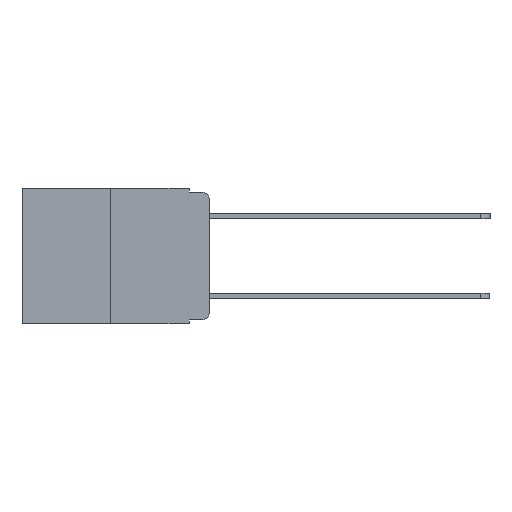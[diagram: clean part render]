
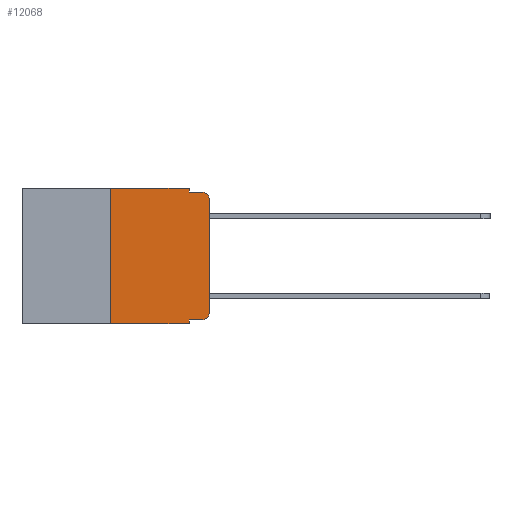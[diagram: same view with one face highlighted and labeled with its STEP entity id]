
A CAD part, left-side view. The second image highlights one B-rep face of the part: STEP entity #12068.
In plain terms, the highlighted planar face has unit normal (-1, 0, 0).
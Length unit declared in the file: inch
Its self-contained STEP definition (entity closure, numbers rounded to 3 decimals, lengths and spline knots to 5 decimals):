
#245 = LINE ( 'NONE', #9016, #10110 ) ;
#717 = VERTEX_POINT ( 'NONE', #9515 ) ;
#1064 = CARTESIAN_POINT ( 'NONE',  ( 0., 0.051, -0.333 ) ) ;
#1111 = CARTESIAN_POINT ( 'NONE',  ( 0., 0.02, -0.333 ) ) ;
#1206 = CARTESIAN_POINT ( 'NONE',  ( 0., 0., -0.313 ) ) ;
#1420 = CARTESIAN_POINT ( 'NONE',  ( 0., 0.051, -0.333 ) ) ;
#1492 = VERTEX_POINT ( 'NONE', #8866 ) ;
#1493 = VERTEX_POINT ( 'NONE', #11662 ) ;
#1680 = CARTESIAN_POINT ( 'NONE',  ( 0., 0.473, 0. ) ) ;
#1775 = EDGE_CURVE ( 'NONE', #717, #7980, #5963, .T. ) ;
#1784 = ORIENTED_EDGE ( 'NONE', *, *, #9876, .F. ) ;
#1862 = AXIS2_PLACEMENT_3D ( 'NONE', #8864, #3312, #9811 ) ;
#1883 = ORIENTED_EDGE ( 'NONE', *, *, #3995, .T. ) ;
#2166 = ORIENTED_EDGE ( 'NONE', *, *, #8312, .T. ) ;
#2198 = ORIENTED_EDGE ( 'NONE', *, *, #6837, .T. ) ;
#2695 = DIRECTION ( 'NONE',  ( 0., 0., -1. ) ) ;
#2985 = ORIENTED_EDGE ( 'NONE', *, *, #1775, .F. ) ;
#2997 = LINE ( 'NONE', #11724, #7945 ) ;
#3125 = CIRCLE ( 'NONE', #7545, 0.02 ) ;
#3213 = CARTESIAN_POINT ( 'NONE',  ( 0., 0.25, -0.343 ) ) ;
#3312 = DIRECTION ( 'NONE',  ( -1., 0., 0. ) ) ;
#3526 = VERTEX_POINT ( 'NONE', #1206 ) ;
#3560 = VECTOR ( 'NONE', #8681, 39.37008 ) ;
#3582 = EDGE_CURVE ( 'NONE', #1493, #1492, #6898, .T. ) ;
#3733 = EDGE_CURVE ( 'NONE', #7812, #717, #245, .T. ) ;
#3995 = EDGE_CURVE ( 'NONE', #4111, #3526, #3125, .T. ) ;
#4086 = VERTEX_POINT ( 'NONE', #1064 ) ;
#4111 = VERTEX_POINT ( 'NONE', #1111 ) ;
#4490 = ORIENTED_EDGE ( 'NONE', *, *, #10609, .F. ) ;
#4678 = CARTESIAN_POINT ( 'NONE',  ( 0., 0.051, 0. ) ) ;
#4817 = EDGE_LOOP ( 'NONE', ( #5367, #6202, #1784, #2985, #10118, #10994, #2198, #4490, #2166, #1883 ) ) ;
#4848 = CARTESIAN_POINT ( 'NONE',  ( 0., 0.02, -0.313 ) ) ;
#5244 = CARTESIAN_POINT ( 'NONE',  ( 0., 0.051, -0.343 ) ) ;
#5331 = DIRECTION ( 'NONE',  ( 0., -1., 0. ) ) ;
#5367 = ORIENTED_EDGE ( 'NONE', *, *, #7205, .T. ) ;
#5391 = VECTOR ( 'NONE', #9935, 39.37008 ) ;
#5682 = LINE ( 'NONE', #1420, #5391 ) ;
#5709 = LINE ( 'NONE', #7772, #3560 ) ;
#5772 = DIRECTION ( 'NONE',  ( 0., 0., -1. ) ) ;
#5963 = LINE ( 'NONE', #4678, #10893 ) ;
#6181 = DIRECTION ( 'NONE',  ( 0., 0., -1. ) ) ;
#6202 = ORIENTED_EDGE ( 'NONE', *, *, #3582, .T. ) ;
#6258 = AXIS2_PLACEMENT_3D ( 'NONE', #1680, #8285, #2695 ) ;
#6389 = EDGE_CURVE ( 'NONE', #10520, #7812, #11910, .T. ) ;
#6538 = LINE ( 'NONE', #7279, #8753 ) ;
#6656 = DIRECTION ( 'NONE',  ( 0., -1., 0. ) ) ;
#6837 = EDGE_CURVE ( 'NONE', #10520, #10619, #6538, .T. ) ;
#6898 = CIRCLE ( 'NONE', #1862, 0.02 ) ;
#7078 = LINE ( 'NONE', #9426, #11728 ) ;
#7205 = EDGE_CURVE ( 'NONE', #3526, #1493, #5709, .T. ) ;
#7279 = CARTESIAN_POINT ( 'NONE',  ( 0., 0.473, -0.343 ) ) ;
#7333 = PLANE ( 'NONE',  #6258 ) ;
#7545 = AXIS2_PLACEMENT_3D ( 'NONE', #4848, #11332, #5772 ) ;
#7592 = CARTESIAN_POINT ( 'NONE',  ( 0., 0.051, -0.01 ) ) ;
#7748 = DIRECTION ( 'NONE',  ( 0., 0., 1. ) ) ;
#7772 = CARTESIAN_POINT ( 'NONE',  ( 0., 0., 0. ) ) ;
#7812 = VERTEX_POINT ( 'NONE', #8349 ) ;
#7945 = VECTOR ( 'NONE', #6181, 39.37008 ) ;
#7980 = VERTEX_POINT ( 'NONE', #7592 ) ;
#8285 = DIRECTION ( 'NONE',  ( 1., 0., 0. ) ) ;
#8312 = EDGE_CURVE ( 'NONE', #4086, #4111, #5682, .T. ) ;
#8349 = CARTESIAN_POINT ( 'NONE',  ( 0., 0.25, 0. ) ) ;
#8371 = DIRECTION ( 'NONE',  ( 0., 0., -1. ) ) ;
#8681 = DIRECTION ( 'NONE',  ( 0., 0., 1. ) ) ;
#8753 = VECTOR ( 'NONE', #11907, 39.37008 ) ;
#8864 = CARTESIAN_POINT ( 'NONE',  ( 0., 0.02, -0.03 ) ) ;
#8866 = CARTESIAN_POINT ( 'NONE',  ( 0., 0.02, -0.01 ) ) ;
#9016 = CARTESIAN_POINT ( 'NONE',  ( 0., 0.473, 0. ) ) ;
#9426 = CARTESIAN_POINT ( 'NONE',  ( 0., 0.051, -0.01 ) ) ;
#9457 = VECTOR ( 'NONE', #7748, 39.37008 ) ;
#9515 = CARTESIAN_POINT ( 'NONE',  ( 0., 0.051, 0. ) ) ;
#9581 = CARTESIAN_POINT ( 'NONE',  ( 0., 0.25, 0. ) ) ;
#9811 = DIRECTION ( 'NONE',  ( 0., 0., -1. ) ) ;
#9876 = EDGE_CURVE ( 'NONE', #7980, #1492, #7078, .T. ) ;
#9935 = DIRECTION ( 'NONE',  ( 0., -1., 0. ) ) ;
#10110 = VECTOR ( 'NONE', #5331, 39.37008 ) ;
#10118 = ORIENTED_EDGE ( 'NONE', *, *, #3733, .F. ) ;
#10520 = VERTEX_POINT ( 'NONE', #3213 ) ;
#10609 = EDGE_CURVE ( 'NONE', #4086, #10619, #2997, .T. ) ;
#10619 = VERTEX_POINT ( 'NONE', #5244 ) ;
#10893 = VECTOR ( 'NONE', #8371, 39.37008 ) ;
#10994 = ORIENTED_EDGE ( 'NONE', *, *, #6389, .F. ) ;
#11332 = DIRECTION ( 'NONE',  ( -1., 0., 0. ) ) ;
#11662 = CARTESIAN_POINT ( 'NONE',  ( 0., 0., -0.03 ) ) ;
#11724 = CARTESIAN_POINT ( 'NONE',  ( 0., 0.051, 0. ) ) ;
#11728 = VECTOR ( 'NONE', #6656, 39.37008 ) ;
#11907 = DIRECTION ( 'NONE',  ( 0., -1., 0. ) ) ;
#11910 = LINE ( 'NONE', #9581, #9457 ) ;
#11939 = FACE_OUTER_BOUND ( 'NONE', #4817, .T. ) ;
#12068 = ADVANCED_FACE ( 'NONE', ( #11939 ), #7333, .F. ) ;
